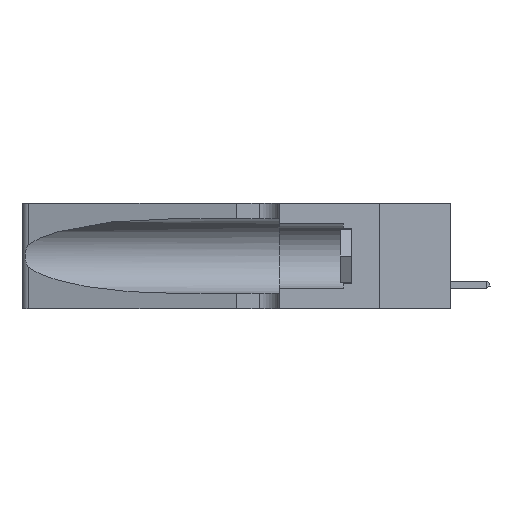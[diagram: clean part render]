
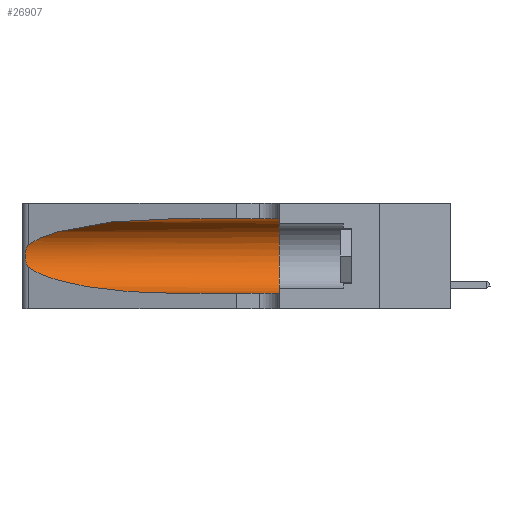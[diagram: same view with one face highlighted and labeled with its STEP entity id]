
A CAD part, left-side view. The second image highlights one B-rep face of the part: STEP entity #26907.
In plain terms, the highlighted cylindrical face has radius 3.308 mm (diameter 6.617 mm), a partial arc.
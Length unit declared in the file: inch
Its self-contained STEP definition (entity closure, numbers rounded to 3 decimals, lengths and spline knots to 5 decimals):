
#88 = VECTOR ( 'NONE', #8485, 39.37008 ) ;
#245 = CARTESIAN_POINT ( 'NONE',  ( 0.25856, 1.23593, 0.16098 ) ) ;
#1174 = EDGE_CURVE ( 'NONE', #10959, #8525, #28769, .T. ) ;
#1817 = CARTESIAN_POINT ( 'NONE',  ( 0.1305, 1.61858, 0.185 ) ) ;
#2178 = EDGE_CURVE ( 'NONE', #8525, #13759, #9660, .T. ) ;
#2518 = ORIENTED_EDGE ( 'NONE', *, *, #5148, .T. ) ;
#2575 = CARTESIAN_POINT ( 'NONE',  ( 0.1305, 0.35, 0.31525 ) ) ;
#3933 = EDGE_CURVE ( 'NONE', #10959, #11572, #23516, .T. ) ;
#4279 = DIRECTION ( 'NONE',  ( 0., -1., 0. ) ) ;
#5148 = EDGE_CURVE ( 'NONE', #24255, #25775, #24457, .T. ) ;
#5852 = CARTESIAN_POINT ( 'NONE',  ( 0.25487, 1.22718, 0.14631 ) ) ;
#7203 = CARTESIAN_POINT ( 'NONE',  ( 0.25639, 1.23186, 0.15144 ) ) ;
#7822 = ORIENTED_EDGE ( 'NONE', *, *, #3933, .T. ) ;
#7921 = EDGE_CURVE ( 'NONE', #25775, #13759, #19576, .T. ) ;
#7990 = CARTESIAN_POINT ( 'NONE',  ( 0.1305, 0.72297, 0.31525 ) ) ;
#8485 = DIRECTION ( 'NONE',  ( 0., -1., 0. ) ) ;
#8525 = VERTEX_POINT ( 'NONE', #2575 ) ;
#8958 = FACE_OUTER_BOUND ( 'NONE', #11048, .T. ) ;
#9415 = CARTESIAN_POINT ( 'NONE',  ( 0.26018, 1.23835, 0.19895 ) ) ;
#9660 = CIRCLE ( 'NONE', #16252, 0.13025 ) ;
#10817 = DIRECTION ( 'NONE',  ( 0., 1., 0. ) ) ;
#10959 = VERTEX_POINT ( 'NONE', #7990 ) ;
#11048 = EDGE_LOOP ( 'NONE', ( #7822, #28486, #2518, #18861, #24732, #25901 ) ) ;
#11543 = CARTESIAN_POINT ( 'NONE',  ( 0.25789, 1.23486, 0.15765 ) ) ;
#11572 = VERTEX_POINT ( 'NONE', #17626 ) ;
#11952 = CARTESIAN_POINT ( 'NONE',  ( 0.26075, 1.23896, 0.19203 ) ) ;
#12256 = CARTESIAN_POINT ( 'NONE',  ( 0.25487, 1.22718, 0.14631 ) ) ;
#12919 = CARTESIAN_POINT ( 'NONE',  ( 0.18966, 0.96281, 0.31525 ) ) ;
#13247 = CARTESIAN_POINT ( 'NONE',  ( 0.2373, 1.15595, 0.08982 ) ) ;
#13252 = CARTESIAN_POINT ( 'NONE',  ( 0.1305, 0.35, 0.185 ) ) ;
#13759 = VERTEX_POINT ( 'NONE', #17981 ) ;
#13774 = VECTOR ( 'NONE', #29932, 39.37008 ) ;
#14007 = CARTESIAN_POINT ( 'NONE',  ( 0.26017, 1.23833, 0.17102 ) ) ;
#14302 = CARTESIAN_POINT ( 'NONE',  ( 0.25487, 1.22718, 0.14631 ) ) ;
#15363 = CARTESIAN_POINT ( 'NONE',  ( 0.2373, 1.15595, 0.28018 ) ) ;
#16228 = CARTESIAN_POINT ( 'NONE',  ( 0.25854, 1.2359, 0.20912 ) ) ;
#16252 = AXIS2_PLACEMENT_3D ( 'NONE', #13252, #10817, #19936 ) ;
#16330 = CARTESIAN_POINT ( 'NONE',  ( 0.25555, 1.22994, 0.2215 ) ) ;
#16517 = CARTESIAN_POINT ( 'NONE',  ( 0.25555, 1.22993, 0.14849 ) ) ;
#17626 = CARTESIAN_POINT ( 'NONE',  ( 0.25487, 1.22718, 0.22369 ) ) ;
#17981 = CARTESIAN_POINT ( 'NONE',  ( 0.1305, 0.35, 0.05475 ) ) ;
#18861 = ORIENTED_EDGE ( 'NONE', *, *, #7921, .T. ) ;
#19477 = B_SPLINE_CURVE_WITH_KNOTS ( 'NONE', 3,
 ( #27757, #16330, #27945, #28049, #16228, #9415, #11952, #21049, #14007, #245, #11543, #7203, #16517, #14302 ),
 .UNSPECIFIED., .F., .F.,
 ( 4, 2, 2, 2, 2, 2, 4 ),
 ( 0., 0.00027, 0.00053, 0.00107, 0.0016, 0.00187, 0.00214 ),
 .UNSPECIFIED. ) ;
#19576 = LINE ( 'NONE', #27684, #13774 ) ;
#19929 = CARTESIAN_POINT ( 'NONE',  ( 0.18966, 0.96281, 0.05475 ) ) ;
#19936 = DIRECTION ( 'NONE',  ( 0., 0., 1. ) ) ;
#20211 = CARTESIAN_POINT ( 'NONE',  ( 0.1305, 0.72297, 0.31525 ) ) ;
#21049 = CARTESIAN_POINT ( 'NONE',  ( 0.26075, 1.23896, 0.178 ) ) ;
#21471 = CARTESIAN_POINT ( 'NONE',  ( 0.1305, 0.72297, 0.05475 ) ) ;
#22442 = CARTESIAN_POINT ( 'NONE',  ( 0.1305, 1.61858, 0.31525 ) ) ;
#23516 =( BOUNDED_CURVE ( )  B_SPLINE_CURVE ( 3, ( #20211, #12919, #15363, #29533 ),
 .UNSPECIFIED., .F., .F. ) 
 B_SPLINE_CURVE_WITH_KNOTS ( ( 4, 4 ),
 ( 1.5708, 2.84003 ),
 .UNSPECIFIED. ) 
 CURVE ( )  GEOMETRIC_REPRESENTATION_ITEM ( )  RATIONAL_B_SPLINE_CURVE ( ( 1., 0.87, 0.87, 1. ) ) 
 REPRESENTATION_ITEM ( '' )  );
#24190 = EDGE_CURVE ( 'NONE', #11572, #24255, #19477, .T. ) ;
#24255 = VERTEX_POINT ( 'NONE', #12256 ) ;
#24457 =( BOUNDED_CURVE ( )  B_SPLINE_CURVE ( 3, ( #5852, #13247, #19929, #26712 ),
 .UNSPECIFIED., .F., .F. ) 
 B_SPLINE_CURVE_WITH_KNOTS ( ( 4, 4 ),
 ( 3.44316, 4.71239 ),
 .UNSPECIFIED. ) 
 CURVE ( )  GEOMETRIC_REPRESENTATION_ITEM ( )  RATIONAL_B_SPLINE_CURVE ( ( 1., 0.87, 0.87, 1. ) ) 
 REPRESENTATION_ITEM ( '' )  );
#24732 = ORIENTED_EDGE ( 'NONE', *, *, #2178, .F. ) ;
#24902 = CYLINDRICAL_SURFACE ( 'NONE', #26850, 0.13025 ) ;
#25775 = VERTEX_POINT ( 'NONE', #21471 ) ;
#25901 = ORIENTED_EDGE ( 'NONE', *, *, #1174, .F. ) ;
#26712 = CARTESIAN_POINT ( 'NONE',  ( 0.1305, 0.72297, 0.05475 ) ) ;
#26850 = AXIS2_PLACEMENT_3D ( 'NONE', #1817, #4279, #28187 ) ;
#26907 = ADVANCED_FACE ( 'NONE', ( #8958 ), #24902, .F. ) ;
#27684 = CARTESIAN_POINT ( 'NONE',  ( 0.1305, 1.61858, 0.05475 ) ) ;
#27757 = CARTESIAN_POINT ( 'NONE',  ( 0.25487, 1.22718, 0.22369 ) ) ;
#27945 = CARTESIAN_POINT ( 'NONE',  ( 0.25639, 1.23184, 0.21858 ) ) ;
#28049 = CARTESIAN_POINT ( 'NONE',  ( 0.25787, 1.23484, 0.2124 ) ) ;
#28187 = DIRECTION ( 'NONE',  ( 0., 0., -1. ) ) ;
#28486 = ORIENTED_EDGE ( 'NONE', *, *, #24190, .T. ) ;
#28769 = LINE ( 'NONE', #22442, #88 ) ;
#29533 = CARTESIAN_POINT ( 'NONE',  ( 0.25487, 1.22718, 0.22369 ) ) ;
#29932 = DIRECTION ( 'NONE',  ( 0., -1., 0. ) ) ;
